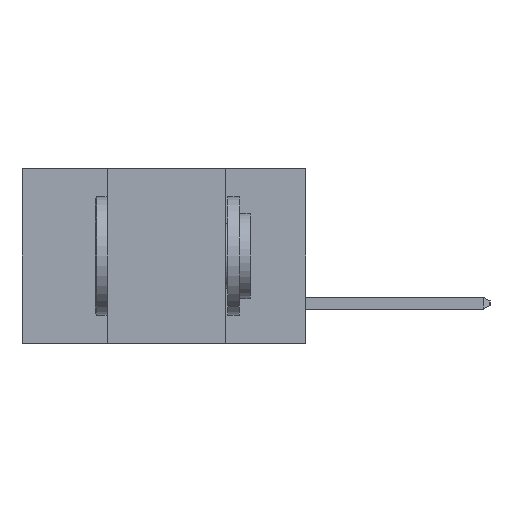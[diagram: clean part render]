
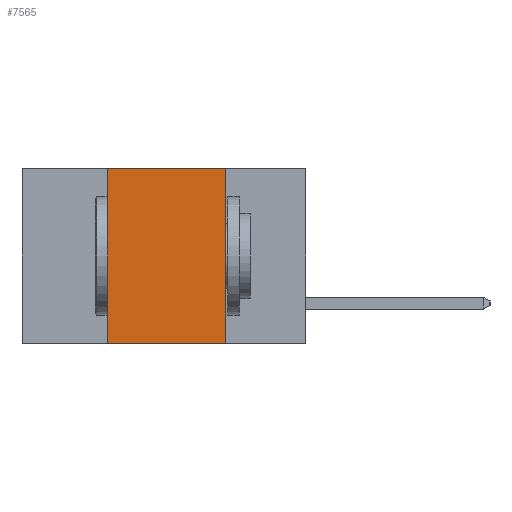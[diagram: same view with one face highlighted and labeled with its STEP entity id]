
A CAD part, left-side view. The second image highlights one B-rep face of the part: STEP entity #7565.
In plain terms, the highlighted planar face has unit normal (-1, 0, 0).
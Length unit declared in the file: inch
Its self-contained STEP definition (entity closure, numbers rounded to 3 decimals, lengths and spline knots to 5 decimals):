
#105 = CARTESIAN_POINT ( 'NONE',  ( 0., 0.17, -0.37 ) ) ;
#191 = FACE_OUTER_BOUND ( 'NONE', #10472, .T. ) ;
#1291 = VERTEX_POINT ( 'NONE', #1372 ) ;
#1362 = DIRECTION ( 'NONE',  ( 0., 0., 1. ) ) ;
#1372 = CARTESIAN_POINT ( 'NONE',  ( 0., 0.17, -0.37 ) ) ;
#1449 = EDGE_CURVE ( 'NONE', #10256, #12750, #1907, .T. ) ;
#1763 = AXIS2_PLACEMENT_3D ( 'NONE', #2864, #2649, #2629 ) ;
#1907 = LINE ( 'NONE', #4836, #14238 ) ;
#2589 = LINE ( 'NONE', #7408, #14902 ) ;
#2629 = DIRECTION ( 'NONE',  ( 0., 0., -1. ) ) ;
#2649 = DIRECTION ( 'NONE',  ( 1., 0., 0. ) ) ;
#2661 = PLANE ( 'NONE',  #1763 ) ;
#2864 = CARTESIAN_POINT ( 'NONE',  ( 0., 0.6, 0. ) ) ;
#3073 = DIRECTION ( 'NONE',  ( 0., -1., 0. ) ) ;
#3282 = CARTESIAN_POINT ( 'NONE',  ( 0., 0.6, -0.37 ) ) ;
#3458 = LINE ( 'NONE', #105, #9858 ) ;
#3835 = ORIENTED_EDGE ( 'NONE', *, *, #5845, .F. ) ;
#4155 = ORIENTED_EDGE ( 'NONE', *, *, #1449, .F. ) ;
#4319 = ORIENTED_EDGE ( 'NONE', *, *, #15330, .F. ) ;
#4528 = ORIENTED_EDGE ( 'NONE', *, *, #4944, .T. ) ;
#4836 = CARTESIAN_POINT ( 'NONE',  ( 0., 0.6, 0. ) ) ;
#4944 = EDGE_CURVE ( 'NONE', #10816, #1291, #5778, .T. ) ;
#5591 = DIRECTION ( 'NONE',  ( 0., -1., 0. ) ) ;
#5778 = LINE ( 'NONE', #3282, #14489 ) ;
#5845 = EDGE_CURVE ( 'NONE', #12750, #1291, #3458, .T. ) ;
#6412 = DIRECTION ( 'NONE',  ( 0., 0., -1. ) ) ;
#7408 = CARTESIAN_POINT ( 'NONE',  ( 0., 0.42, -0.37 ) ) ;
#7565 = ADVANCED_FACE ( 'NONE', ( #191 ), #2661, .F. ) ;
#9858 = VECTOR ( 'NONE', #6412, 39.37008 ) ;
#10256 = VERTEX_POINT ( 'NONE', #12918 ) ;
#10472 = EDGE_LOOP ( 'NONE', ( #3835, #4155, #4319, #4528 ) ) ;
#10816 = VERTEX_POINT ( 'NONE', #13800 ) ;
#12750 = VERTEX_POINT ( 'NONE', #14374 ) ;
#12918 = CARTESIAN_POINT ( 'NONE',  ( 0., 0.42, 0. ) ) ;
#13800 = CARTESIAN_POINT ( 'NONE',  ( 0., 0.42, -0.37 ) ) ;
#14238 = VECTOR ( 'NONE', #5591, 39.37008 ) ;
#14374 = CARTESIAN_POINT ( 'NONE',  ( 0., 0.17, 0. ) ) ;
#14489 = VECTOR ( 'NONE', #3073, 39.37008 ) ;
#14902 = VECTOR ( 'NONE', #1362, 39.37008 ) ;
#15330 = EDGE_CURVE ( 'NONE', #10816, #10256, #2589, .T. ) ;
